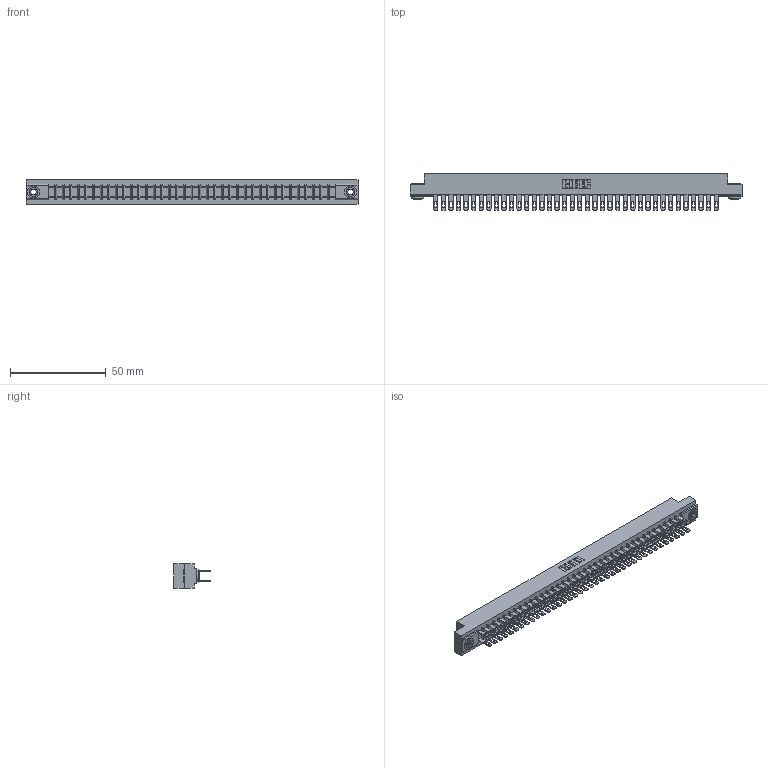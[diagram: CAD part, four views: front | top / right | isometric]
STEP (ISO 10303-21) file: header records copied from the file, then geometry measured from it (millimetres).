
FILE_DESCRIPTION (( 'STEP AP203' ), '1' );
FILE_NAME ('357-076-500-203.STEP', '2019-09-19T13:04:13', ( '' ), ( '' ), 'SwSTEP 2.0', 'SolidWorks 2016', '' );
FILE_SCHEMA (( 'CONFIG_CONTROL_DESIGN' ));
Length unit declared in the file: inch
Products named in the file (4): 345-250-002_345-250-002-102; 357-076-500-203; 307 Part_.156 Dia Mounting Holes; 307-290-001_500
Assembly tree (79 placements, depth 2):
  357-076-500-203
    307 Part_.156 Dia Mounting Holes
    307-290-001_500  x76
    345-250-002_345-250-002-102  x2
Bounding box: 173.58 x 19.18 x 12.7 mm (x, y, z)
Volume: 18649.3 mm3; surface area: 24197.7 mm2
Topology: 79 solids, 79 shells, 3705 faces, 10315 edges, 6666 vertices
Faces by surface type: plane 2374, cylinder 1245, sphere 78, cone 8
Entity records: 35325 total; most frequent: CARTESIAN_POINT 5759, ORIENTED_EDGE 5698, DIRECTION 5659, EDGE_CURVE 2849, LINE 2175, VECTOR 2175, VERTEX_POINT 1842, AXIS2_PLACEMENT_3D 1742
